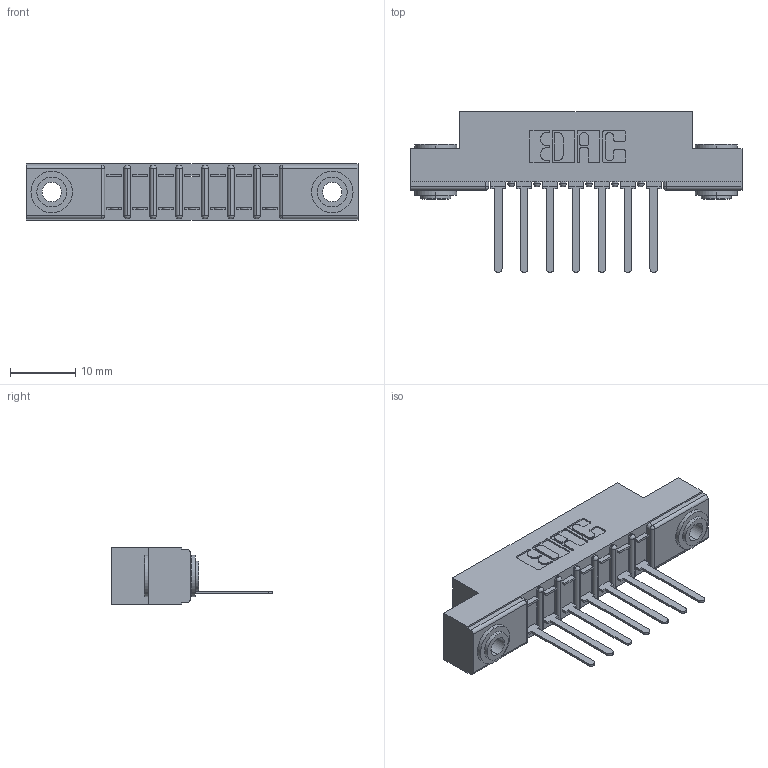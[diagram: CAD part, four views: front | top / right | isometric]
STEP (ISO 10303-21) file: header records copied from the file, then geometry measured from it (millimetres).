
FILE_DESCRIPTION (( 'STEP AP203' ), '1' );
FILE_NAME ('357-007-541-103.STEP', '2018-08-07T00:08:02', ( '' ), ( '' ), 'SwSTEP 2.0', 'SolidWorks 2016', '' );
FILE_SCHEMA (( 'CONFIG_CONTROL_DESIGN' ));
Length unit declared in the file: inch
Products named in the file (4): 345-250-002_345-250-002-102; 357-007-541-103; 307 Part_.156 Dia Mounting Holes; 307-290-002_541
Assembly tree (10 placements, depth 2):
  357-007-541-103
    307 Part_.156 Dia Mounting Holes
    307-290-002_541  x7
    345-250-002_345-250-002-102  x2
Bounding box: 50.75 x 24.59 x 8.71 mm (x, y, z)
Volume: 3363.6 mm3; surface area: 5647 mm2
Topology: 10 solids, 10 shells, 696 faces, 2059 edges, 1346 vertices
Faces by surface type: plane 409, cylinder 263, sphere 16, cone 8
Entity records: 12099 total; most frequent: CARTESIAN_POINT 2013, ORIENTED_EDGE 1994, DIRECTION 1987, EDGE_CURVE 997, VECTOR 739, LINE 739, VERTEX_POINT 650, AXIS2_PLACEMENT_3D 624
